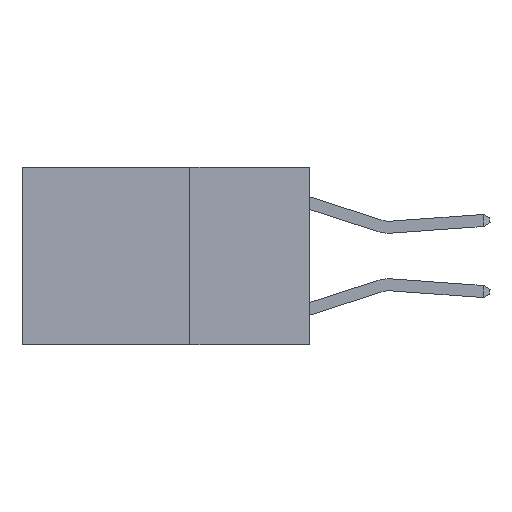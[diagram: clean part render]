
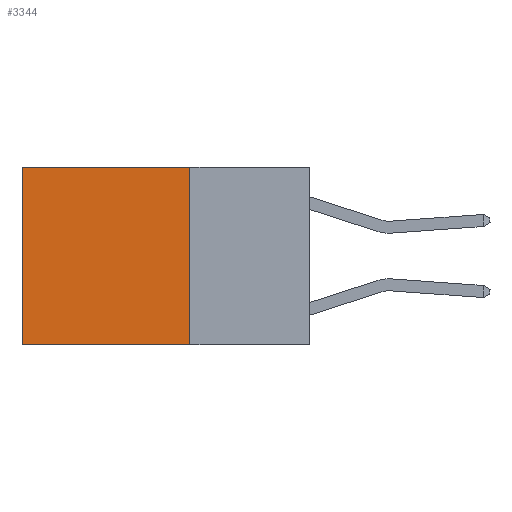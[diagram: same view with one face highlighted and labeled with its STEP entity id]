
A CAD part, left-side view. The second image highlights one B-rep face of the part: STEP entity #3344.
In plain terms, the highlighted planar face has unit normal (-1, 0, 0).
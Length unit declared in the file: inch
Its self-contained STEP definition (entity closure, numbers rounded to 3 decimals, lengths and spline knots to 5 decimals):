
#502 = EDGE_CURVE ( 'NONE', #9265, #4522, #13642, .T. ) ;
#1448 = LINE ( 'NONE', #8955, #7985 ) ;
#1951 = PLANE ( 'NONE',  #5189 ) ;
#2009 = ORIENTED_EDGE ( 'NONE', *, *, #502, .F. ) ;
#2027 = VECTOR ( 'NONE', #2768, 39.37008 ) ;
#2354 = DIRECTION ( 'NONE',  ( 0., 0., -1. ) ) ;
#2768 = DIRECTION ( 'NONE',  ( 0., 0., -1. ) ) ;
#2874 = LINE ( 'NONE', #9526, #2912 ) ;
#2912 = VECTOR ( 'NONE', #7234, 39.37008 ) ;
#3072 = FACE_OUTER_BOUND ( 'NONE', #10768, .T. ) ;
#3214 = DIRECTION ( 'NONE',  ( 1., 0., 0. ) ) ;
#3344 = ADVANCED_FACE ( 'NONE', ( #3072 ), #1951, .F. ) ;
#3982 = CARTESIAN_POINT ( 'NONE',  ( 0.2625, 0.6, 0. ) ) ;
#4069 = DIRECTION ( 'NONE',  ( 0., 0., -1. ) ) ;
#4394 = ORIENTED_EDGE ( 'NONE', *, *, #7104, .F. ) ;
#4522 = VERTEX_POINT ( 'NONE', #12145 ) ;
#5189 = AXIS2_PLACEMENT_3D ( 'NONE', #11738, #3214, #4069 ) ;
#5687 = ORIENTED_EDGE ( 'NONE', *, *, #11574, .T. ) ;
#6123 = VERTEX_POINT ( 'NONE', #13926 ) ;
#6904 = VECTOR ( 'NONE', #13716, 39.37008 ) ;
#7104 = EDGE_CURVE ( 'NONE', #6123, #9265, #1448, .T. ) ;
#7234 = DIRECTION ( 'NONE',  ( 0., 1., 0. ) ) ;
#7405 = VERTEX_POINT ( 'NONE', #3982 ) ;
#7985 = VECTOR ( 'NONE', #2354, 39.37008 ) ;
#8955 = CARTESIAN_POINT ( 'NONE',  ( 0.2625, 0.25, 0. ) ) ;
#9265 = VERTEX_POINT ( 'NONE', #11968 ) ;
#9493 = CARTESIAN_POINT ( 'NONE',  ( 0.2625, 0.25, -0.37 ) ) ;
#9526 = CARTESIAN_POINT ( 'NONE',  ( 0.2625, 0.25, 0. ) ) ;
#9910 = ORIENTED_EDGE ( 'NONE', *, *, #13832, .T. ) ;
#10768 = EDGE_LOOP ( 'NONE', ( #5687, #2009, #4394, #9910 ) ) ;
#11574 = EDGE_CURVE ( 'NONE', #7405, #4522, #12493, .T. ) ;
#11738 = CARTESIAN_POINT ( 'NONE',  ( 0.2625, 0.25, 0. ) ) ;
#11968 = CARTESIAN_POINT ( 'NONE',  ( 0.2625, 0.25, -0.37 ) ) ;
#12145 = CARTESIAN_POINT ( 'NONE',  ( 0.2625, 0.6, -0.37 ) ) ;
#12426 = CARTESIAN_POINT ( 'NONE',  ( 0.2625, 0.6, 0. ) ) ;
#12493 = LINE ( 'NONE', #12426, #2027 ) ;
#13642 = LINE ( 'NONE', #9493, #6904 ) ;
#13716 = DIRECTION ( 'NONE',  ( 0., 1., 0. ) ) ;
#13832 = EDGE_CURVE ( 'NONE', #6123, #7405, #2874, .T. ) ;
#13926 = CARTESIAN_POINT ( 'NONE',  ( 0.2625, 0.25, 0. ) ) ;
